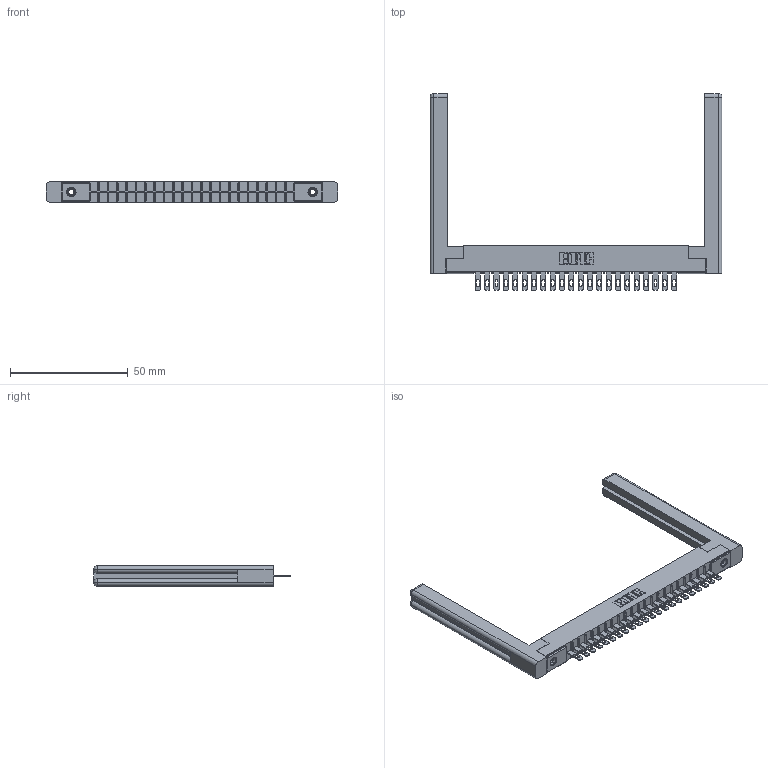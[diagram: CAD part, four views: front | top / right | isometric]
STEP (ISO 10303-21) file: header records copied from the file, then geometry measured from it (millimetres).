
FILE_DESCRIPTION (( 'STEP AP203' ), '1' );
FILE_NAME ('306-022-400-158.STEP', '2020-09-21T21:13:23', ( '' ), ( '' ), 'SwSTEP 2.0', 'SolidWorks 2020', '' );
FILE_SCHEMA (( 'CONFIG_CONTROL_DESIGN' ));
Length unit declared in the file: inch
Products named in the file (5): 306-022-400-158; 345-250-001_345-250-001-102; 307-220-058; 306-290-001_100; 306 Part_.156 Dia
Assembly tree (27 placements, depth 2):
  306-022-400-158
    306 Part_.156 Dia
    306-290-001_100  x22
    345-250-001_345-250-001-102  x2
    307-220-058  x2
Bounding box: 123.8 x 83.52 x 8.71 mm (x, y, z)
Volume: 16179.7 mm3; surface area: 18267.2 mm2
Topology: 27 solids, 27 shells, 1930 faces, 5400 edges, 3468 vertices
Faces by surface type: plane 1252, cylinder 566, sphere 88, cone 12, torus 12
Entity records: 25904 total; most frequent: CARTESIAN_POINT 4356, ORIENTED_EDGE 4258, DIRECTION 4253, EDGE_CURVE 2129, VECTOR 1647, LINE 1647, VERTEX_POINT 1352, AXIS2_PLACEMENT_3D 1303
